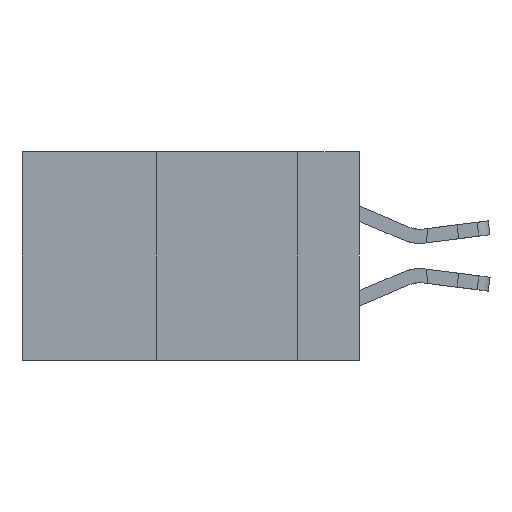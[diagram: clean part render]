
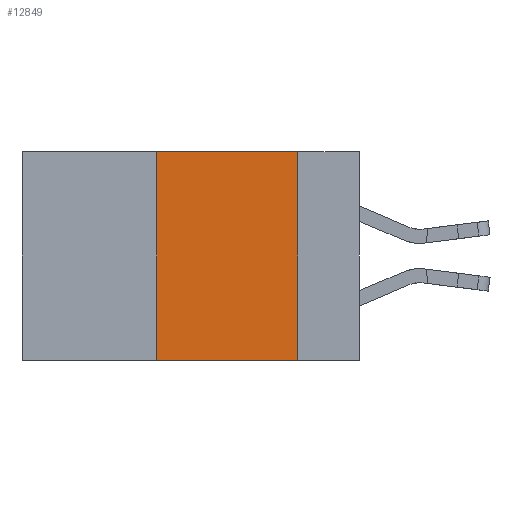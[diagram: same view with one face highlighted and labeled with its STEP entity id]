
A CAD part, left-side view. The second image highlights one B-rep face of the part: STEP entity #12849.
In plain terms, the highlighted planar face has unit normal (-1, 0, 0).
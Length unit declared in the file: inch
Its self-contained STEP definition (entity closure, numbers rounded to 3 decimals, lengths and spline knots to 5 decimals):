
#304 = CARTESIAN_POINT ( 'NONE',  ( 0., 0.6, -0.37 ) ) ;
#835 = FACE_OUTER_BOUND ( 'NONE', #15514, .T. ) ;
#1985 = DIRECTION ( 'NONE',  ( 0., -1., 0. ) ) ;
#2873 = AXIS2_PLACEMENT_3D ( 'NONE', #9714, #7325, #16148 ) ;
#3045 = LINE ( 'NONE', #10469, #11790 ) ;
#4012 = ORIENTED_EDGE ( 'NONE', *, *, #8731, .F. ) ;
#4624 = CARTESIAN_POINT ( 'NONE',  ( 0., 0.6, 0. ) ) ;
#4707 = LINE ( 'NONE', #304, #5874 ) ;
#5014 = DIRECTION ( 'NONE',  ( 0., 0., -1. ) ) ;
#5468 = ORIENTED_EDGE ( 'NONE', *, *, #11449, .F. ) ;
#5538 = DIRECTION ( 'NONE',  ( 0., -1., 0. ) ) ;
#5874 = VECTOR ( 'NONE', #5538, 39.37008 ) ;
#6895 = VERTEX_POINT ( 'NONE', #15695 ) ;
#7325 = DIRECTION ( 'NONE',  ( 1., 0., 0. ) ) ;
#7470 = VECTOR ( 'NONE', #5014, 39.37008 ) ;
#7907 = CARTESIAN_POINT ( 'NONE',  ( 0., 0.11, 0. ) ) ;
#8731 = EDGE_CURVE ( 'NONE', #15972, #15655, #10813, .T. ) ;
#9714 = CARTESIAN_POINT ( 'NONE',  ( 0., 0.6, 0. ) ) ;
#10094 = LINE ( 'NONE', #4624, #10667 ) ;
#10469 = CARTESIAN_POINT ( 'NONE',  ( 0., 0.36, 0. ) ) ;
#10667 = VECTOR ( 'NONE', #1985, 39.37008 ) ;
#10813 = LINE ( 'NONE', #7907, #7470 ) ;
#10877 = VERTEX_POINT ( 'NONE', #11596 ) ;
#11068 = PLANE ( 'NONE',  #2873 ) ;
#11449 = EDGE_CURVE ( 'NONE', #10877, #15972, #10094, .T. ) ;
#11596 = CARTESIAN_POINT ( 'NONE',  ( 0., 0.36, 0. ) ) ;
#11790 = VECTOR ( 'NONE', #14077, 39.37008 ) ;
#12336 = CARTESIAN_POINT ( 'NONE',  ( 0., 0.11, -0.37 ) ) ;
#12849 = ADVANCED_FACE ( 'NONE', ( #835 ), #11068, .F. ) ;
#13621 = CARTESIAN_POINT ( 'NONE',  ( 0., 0.11, 0. ) ) ;
#13663 = EDGE_CURVE ( 'NONE', #6895, #15655, #4707, .T. ) ;
#14077 = DIRECTION ( 'NONE',  ( 0., 0., 1. ) ) ;
#14552 = EDGE_CURVE ( 'NONE', #6895, #10877, #3045, .T. ) ;
#14595 = ORIENTED_EDGE ( 'NONE', *, *, #14552, .F. ) ;
#15514 = EDGE_LOOP ( 'NONE', ( #4012, #5468, #14595, #16305 ) ) ;
#15655 = VERTEX_POINT ( 'NONE', #12336 ) ;
#15695 = CARTESIAN_POINT ( 'NONE',  ( 0., 0.36, -0.37 ) ) ;
#15972 = VERTEX_POINT ( 'NONE', #13621 ) ;
#16148 = DIRECTION ( 'NONE',  ( 0., 0., -1. ) ) ;
#16305 = ORIENTED_EDGE ( 'NONE', *, *, #13663, .T. ) ;
